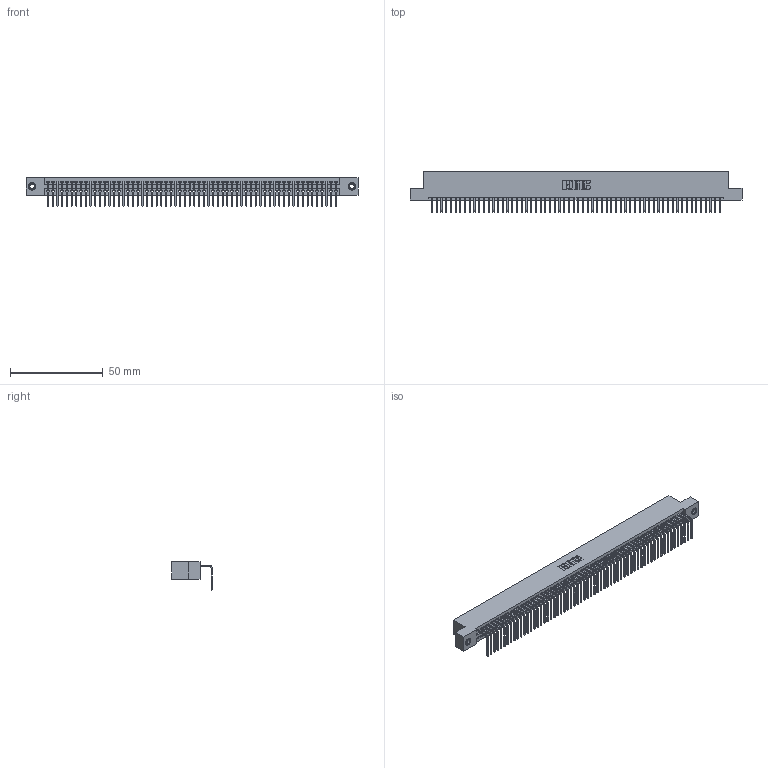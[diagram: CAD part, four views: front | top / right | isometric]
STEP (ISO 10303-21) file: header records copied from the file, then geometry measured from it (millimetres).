
FILE_DESCRIPTION (( 'STEP AP203' ), '1' );
FILE_NAME ('395-062-558-107.STEP', '2018-11-24T05:22:41', ( '' ), ( '' ), 'SwSTEP 2.0', 'SolidWorks 2016', '' );
FILE_SCHEMA (( 'CONFIG_CONTROL_DESIGN' ));
Length unit declared in the file: inch
Products named in the file (4): 345 Part_Flush Mounting Lugs - 0.156 Dia-TI; 345-292-001_558 Tail - 2; 395-062-558-107; 345-250-001_345-250-005-103
Assembly tree (65 placements, depth 2):
  395-062-558-107
    345 Part_Flush Mounting Lugs - 0.156 Dia-TI
    345-292-001_558 Tail - 2  x62
    345-250-001_345-250-005-103  x2
Bounding box: 178.69 x 21.83 x 15.37 mm (x, y, z)
Volume: 17329 mm3; surface area: 24546.8 mm2
Topology: 65 solids, 65 shells, 3906 faces, 11761 edges, 7750 vertices
Faces by surface type: plane 2716, cylinder 1174, cone 12, torus 4
Entity records: 45240 total; most frequent: CARTESIAN_POINT 7817, ORIENTED_EDGE 7806, DIRECTION 6825, EDGE_CURVE 3903, LINE 3503, VECTOR 3503, VERTEX_POINT 2596, AXIS2_PLACEMENT_3D 1661
